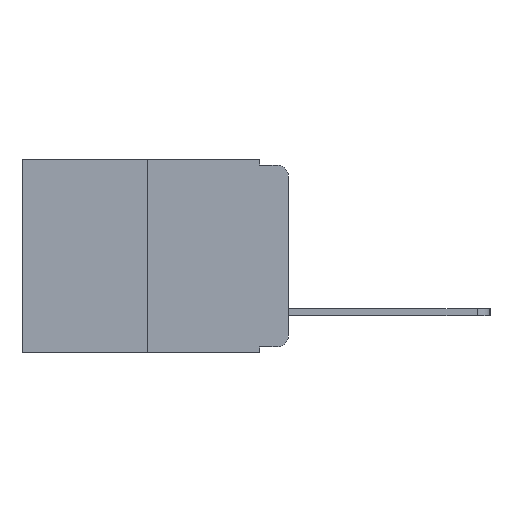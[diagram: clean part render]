
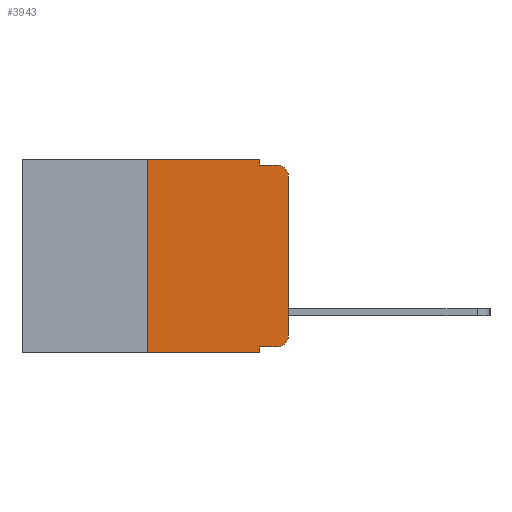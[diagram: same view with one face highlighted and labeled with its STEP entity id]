
A CAD part, left-side view. The second image highlights one B-rep face of the part: STEP entity #3943.
In plain terms, the highlighted planar face has unit normal (-1, 0, 0).
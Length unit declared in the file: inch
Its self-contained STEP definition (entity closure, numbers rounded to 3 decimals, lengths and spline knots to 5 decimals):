
#148 = EDGE_CURVE ( 'NONE', #6284, #319, #4667, .T. ) ;
#247 = ORIENTED_EDGE ( 'NONE', *, *, #1175, .F. ) ;
#298 = ORIENTED_EDGE ( 'NONE', *, *, #7381, .F. ) ;
#319 = VERTEX_POINT ( 'NONE', #2803 ) ;
#545 = LINE ( 'NONE', #9095, #3030 ) ;
#684 = ORIENTED_EDGE ( 'NONE', *, *, #4936, .T. ) ;
#885 = ORIENTED_EDGE ( 'NONE', *, *, #8469, .T. ) ;
#894 = ORIENTED_EDGE ( 'NONE', *, *, #148, .F. ) ;
#1029 = VERTEX_POINT ( 'NONE', #1337 ) ;
#1103 = VERTEX_POINT ( 'NONE', #2449 ) ;
#1175 = EDGE_CURVE ( 'NONE', #8988, #1029, #6311, .T. ) ;
#1337 = CARTESIAN_POINT ( 'NONE',  ( 0., 0.02, -0.01 ) ) ;
#1626 = VECTOR ( 'NONE', #4098, 39.37008 ) ;
#1685 = EDGE_CURVE ( 'NONE', #1103, #319, #545, .T. ) ;
#1698 = DIRECTION ( 'NONE',  ( 0., 0., 1. ) ) ;
#1765 = AXIS2_PLACEMENT_3D ( 'NONE', #1854, #1932, #1923 ) ;
#1824 = EDGE_CURVE ( 'NONE', #1103, #1863, #3461, .T. ) ;
#1854 = CARTESIAN_POINT ( 'NONE',  ( 0., 0.02, -0.03 ) ) ;
#1861 = EDGE_LOOP ( 'NONE', ( #4172, #4598, #247, #2723, #298, #3576, #2765, #894, #885, #684 ) ) ;
#1863 = VERTEX_POINT ( 'NONE', #2095 ) ;
#1923 = DIRECTION ( 'NONE',  ( 0., 0., -1. ) ) ;
#1932 = DIRECTION ( 'NONE',  ( -1., 0., 0. ) ) ;
#2095 = CARTESIAN_POINT ( 'NONE',  ( 0., 0.25, 0. ) ) ;
#2180 = CARTESIAN_POINT ( 'NONE',  ( 0., 0.051, 0. ) ) ;
#2398 = CARTESIAN_POINT ( 'NONE',  ( 0., 0., -0.313 ) ) ;
#2449 = CARTESIAN_POINT ( 'NONE',  ( 0., 0.25, -0.343 ) ) ;
#2723 = ORIENTED_EDGE ( 'NONE', *, *, #6001, .F. ) ;
#2743 = LINE ( 'NONE', #10051, #9060 ) ;
#2765 = ORIENTED_EDGE ( 'NONE', *, *, #1685, .T. ) ;
#2803 = CARTESIAN_POINT ( 'NONE',  ( 0., 0.051, -0.343 ) ) ;
#2816 = AXIS2_PLACEMENT_3D ( 'NONE', #5940, #5979, #6723 ) ;
#2990 = CARTESIAN_POINT ( 'NONE',  ( 0., 0.02, -0.333 ) ) ;
#3030 = VECTOR ( 'NONE', #10559, 39.37008 ) ;
#3167 = DIRECTION ( 'NONE',  ( 0., -1., 0. ) ) ;
#3461 = LINE ( 'NONE', #7890, #7586 ) ;
#3576 = ORIENTED_EDGE ( 'NONE', *, *, #1824, .F. ) ;
#3597 = LINE ( 'NONE', #8459, #5771 ) ;
#3835 = CARTESIAN_POINT ( 'NONE',  ( 0., 0.051, -0.333 ) ) ;
#3943 = ADVANCED_FACE ( 'NONE', ( #9495 ), #6633, .F. ) ;
#4047 = VERTEX_POINT ( 'NONE', #2398 ) ;
#4098 = DIRECTION ( 'NONE',  ( 0., 0., -1. ) ) ;
#4172 = ORIENTED_EDGE ( 'NONE', *, *, #8970, .T. ) ;
#4301 = DIRECTION ( 'NONE',  ( 0., 0., -1. ) ) ;
#4437 = DIRECTION ( 'NONE',  ( -1., 0., 0. ) ) ;
#4503 = AXIS2_PLACEMENT_3D ( 'NONE', #9138, #4437, #4301 ) ;
#4598 = ORIENTED_EDGE ( 'NONE', *, *, #9542, .T. ) ;
#4667 = LINE ( 'NONE', #9303, #6821 ) ;
#4936 = EDGE_CURVE ( 'NONE', #9987, #4047, #10360, .T. ) ;
#5771 = VECTOR ( 'NONE', #9130, 39.37008 ) ;
#5781 = VECTOR ( 'NONE', #10554, 39.37008 ) ;
#5940 = CARTESIAN_POINT ( 'NONE',  ( 0., 0.473, 0. ) ) ;
#5979 = DIRECTION ( 'NONE',  ( 1., 0., 0. ) ) ;
#6001 = EDGE_CURVE ( 'NONE', #9502, #8988, #6462, .T. ) ;
#6219 = VERTEX_POINT ( 'NONE', #9666 ) ;
#6284 = VERTEX_POINT ( 'NONE', #3835 ) ;
#6311 = LINE ( 'NONE', #6620, #9804 ) ;
#6334 = CARTESIAN_POINT ( 'NONE',  ( 0., 0.473, 0. ) ) ;
#6361 = CARTESIAN_POINT ( 'NONE',  ( 0., 0.051, 0. ) ) ;
#6462 = LINE ( 'NONE', #6361, #1626 ) ;
#6620 = CARTESIAN_POINT ( 'NONE',  ( 0., 0.051, -0.01 ) ) ;
#6633 = PLANE ( 'NONE',  #2816 ) ;
#6723 = DIRECTION ( 'NONE',  ( 0., 0., -1. ) ) ;
#6821 = VECTOR ( 'NONE', #7416, 39.37008 ) ;
#7140 = CARTESIAN_POINT ( 'NONE',  ( 0., 0.051, -0.01 ) ) ;
#7381 = EDGE_CURVE ( 'NONE', #1863, #9502, #9789, .T. ) ;
#7416 = DIRECTION ( 'NONE',  ( 0., 0., -1. ) ) ;
#7586 = VECTOR ( 'NONE', #9058, 39.37008 ) ;
#7890 = CARTESIAN_POINT ( 'NONE',  ( 0., 0.25, 0. ) ) ;
#8459 = CARTESIAN_POINT ( 'NONE',  ( 0., 0.051, -0.333 ) ) ;
#8469 = EDGE_CURVE ( 'NONE', #6284, #9987, #3597, .T. ) ;
#8555 = CIRCLE ( 'NONE', #1765, 0.02 ) ;
#8970 = EDGE_CURVE ( 'NONE', #4047, #6219, #2743, .T. ) ;
#8988 = VERTEX_POINT ( 'NONE', #7140 ) ;
#9058 = DIRECTION ( 'NONE',  ( 0., 0., 1. ) ) ;
#9060 = VECTOR ( 'NONE', #1698, 39.37008 ) ;
#9095 = CARTESIAN_POINT ( 'NONE',  ( 0., 0.473, -0.343 ) ) ;
#9130 = DIRECTION ( 'NONE',  ( 0., -1., 0. ) ) ;
#9138 = CARTESIAN_POINT ( 'NONE',  ( 0., 0.02, -0.313 ) ) ;
#9303 = CARTESIAN_POINT ( 'NONE',  ( 0., 0.051, 0. ) ) ;
#9495 = FACE_OUTER_BOUND ( 'NONE', #1861, .T. ) ;
#9502 = VERTEX_POINT ( 'NONE', #2180 ) ;
#9542 = EDGE_CURVE ( 'NONE', #6219, #1029, #8555, .T. ) ;
#9666 = CARTESIAN_POINT ( 'NONE',  ( 0., 0., -0.03 ) ) ;
#9789 = LINE ( 'NONE', #6334, #5781 ) ;
#9804 = VECTOR ( 'NONE', #3167, 39.37008 ) ;
#9987 = VERTEX_POINT ( 'NONE', #2990 ) ;
#10051 = CARTESIAN_POINT ( 'NONE',  ( 0., 0., 0. ) ) ;
#10360 = CIRCLE ( 'NONE', #4503, 0.02 ) ;
#10554 = DIRECTION ( 'NONE',  ( 0., -1., 0. ) ) ;
#10559 = DIRECTION ( 'NONE',  ( 0., -1., 0. ) ) ;
